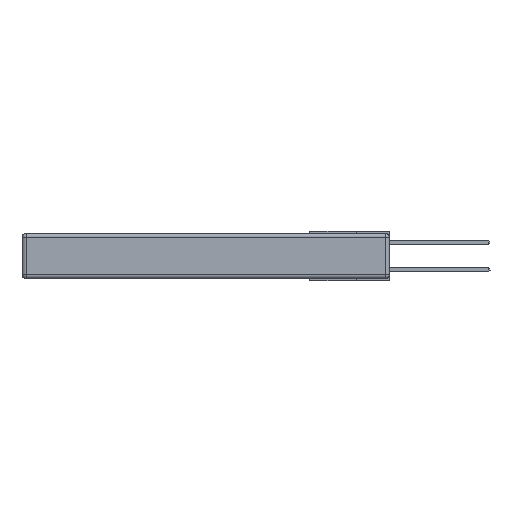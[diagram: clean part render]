
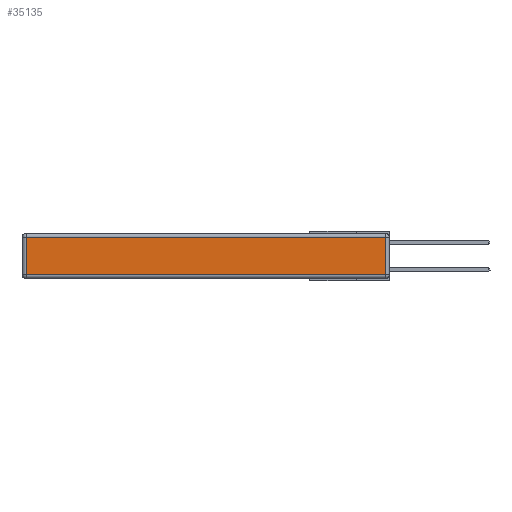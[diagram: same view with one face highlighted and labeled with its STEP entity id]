
A CAD part, left-side view. The second image highlights one B-rep face of the part: STEP entity #35135.
In plain terms, the highlighted planar face has unit normal (-1, 0, 0).
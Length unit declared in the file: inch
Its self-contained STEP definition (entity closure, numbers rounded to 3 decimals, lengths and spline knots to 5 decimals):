
#7 = ORIENTED_EDGE ( 'NONE', *, *, #1794, .T. ) ;
#727 = ORIENTED_EDGE ( 'NONE', *, *, #23576, .T. ) ;
#831 = CARTESIAN_POINT ( 'NONE',  ( 0., 2.72, -0.343 ) ) ;
#1794 = EDGE_CURVE ( 'NONE', #12633, #20697, #6444, .T. ) ;
#5297 = VERTEX_POINT ( 'NONE', #10566 ) ;
#5453 = LINE ( 'NONE', #16434, #18009 ) ;
#6066 = EDGE_LOOP ( 'NONE', ( #727, #34748, #20448, #7 ) ) ;
#6444 = LINE ( 'NONE', #831, #34550 ) ;
#6631 = EDGE_CURVE ( 'NONE', #5297, #29797, #5453, .T. ) ;
#6687 = FACE_OUTER_BOUND ( 'NONE', #6066, .T. ) ;
#8668 = CARTESIAN_POINT ( 'NONE',  ( 0., 0.03, -0.03 ) ) ;
#8839 = LINE ( 'NONE', #10774, #12740 ) ;
#9217 = LINE ( 'NONE', #15573, #21713 ) ;
#10255 = DIRECTION ( 'NONE',  ( 0., 1., 0. ) ) ;
#10566 = CARTESIAN_POINT ( 'NONE',  ( 0., 0.03, -0.313 ) ) ;
#10774 = CARTESIAN_POINT ( 'NONE',  ( 0., 0., -0.313 ) ) ;
#10983 = EDGE_CURVE ( 'NONE', #29797, #12633, #9217, .T. ) ;
#12633 = VERTEX_POINT ( 'NONE', #25863 ) ;
#12740 = VECTOR ( 'NONE', #30242, 39.37008 ) ;
#13973 = CARTESIAN_POINT ( 'NONE',  ( 0., 2.72, -0.313 ) ) ;
#14425 = PLANE ( 'NONE',  #17104 ) ;
#15573 = CARTESIAN_POINT ( 'NONE',  ( 0., 2.75, -0.03 ) ) ;
#16434 = CARTESIAN_POINT ( 'NONE',  ( 0., 0.03, -0.343 ) ) ;
#17104 = AXIS2_PLACEMENT_3D ( 'NONE', #20072, #30964, #33599 ) ;
#18009 = VECTOR ( 'NONE', #24649, 39.37008 ) ;
#20072 = CARTESIAN_POINT ( 'NONE',  ( 0., 0., -0.343 ) ) ;
#20448 = ORIENTED_EDGE ( 'NONE', *, *, #10983, .T. ) ;
#20697 = VERTEX_POINT ( 'NONE', #13973 ) ;
#21713 = VECTOR ( 'NONE', #10255, 39.37008 ) ;
#23576 = EDGE_CURVE ( 'NONE', #20697, #5297, #8839, .T. ) ;
#24649 = DIRECTION ( 'NONE',  ( 0., 0., 1. ) ) ;
#25850 = DIRECTION ( 'NONE',  ( 0., 0., -1. ) ) ;
#25863 = CARTESIAN_POINT ( 'NONE',  ( 0., 2.72, -0.03 ) ) ;
#29797 = VERTEX_POINT ( 'NONE', #8668 ) ;
#30242 = DIRECTION ( 'NONE',  ( 0., -1., 0. ) ) ;
#30964 = DIRECTION ( 'NONE',  ( -1., 0., 0. ) ) ;
#33599 = DIRECTION ( 'NONE',  ( 0., 0., 1. ) ) ;
#34550 = VECTOR ( 'NONE', #25850, 39.37008 ) ;
#34748 = ORIENTED_EDGE ( 'NONE', *, *, #6631, .T. ) ;
#35135 = ADVANCED_FACE ( 'NONE', ( #6687 ), #14425, .T. ) ;
